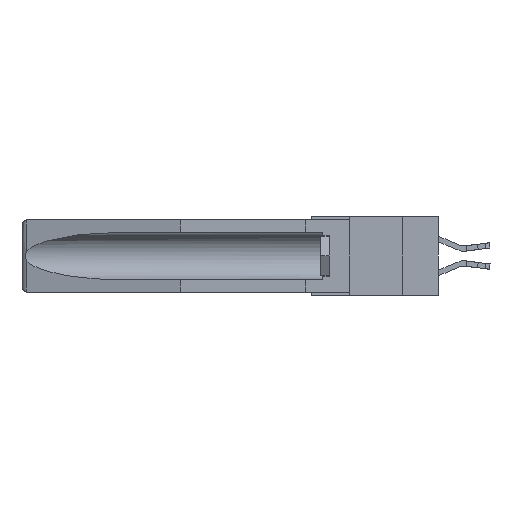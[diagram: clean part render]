
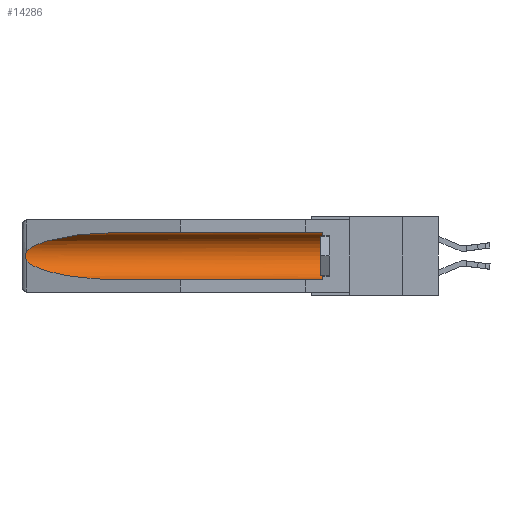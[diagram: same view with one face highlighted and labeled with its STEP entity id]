
A CAD part, left-side view. The second image highlights one B-rep face of the part: STEP entity #14286.
In plain terms, the highlighted cylindrical face has radius 2.857 mm (diameter 5.715 mm), a partial arc.
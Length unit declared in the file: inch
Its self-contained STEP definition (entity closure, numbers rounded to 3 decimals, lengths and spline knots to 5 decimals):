
#65 = LINE ( 'NONE', #9262, #738 ) ;
#738 = VECTOR ( 'NONE', #926, 39.37008 ) ;
#803 = CARTESIAN_POINT ( 'NONE',  ( 0.2673, 1.53269, -0.17917 ) ) ;
#886 = CARTESIAN_POINT ( 'NONE',  ( 0.26654, 1.53092, -0.15636 ) ) ;
#907 = AXIS2_PLACEMENT_3D ( 'NONE', #20044, #23968, #19948 ) ;
#926 = DIRECTION ( 'NONE',  ( 0., 1., 0. ) ) ;
#1354 = VECTOR ( 'NONE', #16719, 39.37008 ) ;
#1902 = CARTESIAN_POINT ( 'NONE',  ( 0.155, -0.30754, -0.284 ) ) ;
#2129 = ORIENTED_EDGE ( 'NONE', *, *, #13327, .T. ) ;
#3458 = CARTESIAN_POINT ( 'NONE',  ( 0.26537, 1.52718, -0.19328 ) ) ;
#3686 = CARTESIAN_POINT ( 'NONE',  ( 0.25451, 1.48313, -0.24835 ) ) ;
#4450 = CARTESIAN_POINT ( 'NONE',  ( 0.155, 1.07973, -0.284 ) ) ;
#4640 = VERTEX_POINT ( 'NONE', #20099 ) ;
#4865 = VERTEX_POINT ( 'NONE', #12742 ) ;
#6241 = EDGE_LOOP ( 'NONE', ( #12499, #10017, #22290, #25767, #2129, #13430 ) ) ;
#6479 = DIRECTION ( 'NONE',  ( 0., 1., 0. ) ) ;
#6636 = VERTEX_POINT ( 'NONE', #12800 ) ;
#6660 = DIRECTION ( 'NONE',  ( 0., 0., 1. ) ) ;
#6828 = CARTESIAN_POINT ( 'NONE',  ( 0.155, 1.07973, -0.059 ) ) ;
#7021 = CARTESIAN_POINT ( 'NONE',  ( 0.26537, 1.52718, -0.14972 ) ) ;
#7631 = VERTEX_POINT ( 'NONE', #4450 ) ;
#7727 = CARTESIAN_POINT ( 'NONE',  ( 0.26537, 1.52718, -0.14972 ) ) ;
#7776 = CARTESIAN_POINT ( 'NONE',  ( 0.21114, 1.30732, -0.284 ) ) ;
#8045 = EDGE_CURVE ( 'NONE', #4865, #6636, #65, .T. ) ;
#9262 = CARTESIAN_POINT ( 'NONE',  ( 0.155, -0.30754, -0.059 ) ) ;
#9271 = FACE_OUTER_BOUND ( 'NONE', #6241, .T. ) ;
#10017 = ORIENTED_EDGE ( 'NONE', *, *, #22010, .T. ) ;
#11835 = CARTESIAN_POINT ( 'NONE',  ( 0.26537, 1.52718, -0.19328 ) ) ;
#12499 = ORIENTED_EDGE ( 'NONE', *, *, #20552, .T. ) ;
#12742 = CARTESIAN_POINT ( 'NONE',  ( 0.155, 0.126, -0.059 ) ) ;
#12800 = CARTESIAN_POINT ( 'NONE',  ( 0.155, 1.07973, -0.059 ) ) ;
#13327 = EDGE_CURVE ( 'NONE', #16865, #4865, #15032, .T. ) ;
#13430 = ORIENTED_EDGE ( 'NONE', *, *, #8045, .T. ) ;
#14097 = CARTESIAN_POINT ( 'NONE',  ( 0.155, 1.07973, -0.284 ) ) ;
#14286 = ADVANCED_FACE ( 'NONE', ( #9271 ), #26576, .F. ) ;
#15032 = CIRCLE ( 'NONE', #907, 0.1125 ) ;
#15741 = LINE ( 'NONE', #1902, #1354 ) ;
#15968 = CARTESIAN_POINT ( 'NONE',  ( 0.26655, 1.53094, -0.18657 ) ) ;
#16456 = CARTESIAN_POINT ( 'NONE',  ( 0.155, 0.126, -0.284 ) ) ;
#16618 =( BOUNDED_CURVE ( )  B_SPLINE_CURVE ( 3, ( #11835, #3686, #7776, #14097 ),
 .UNSPECIFIED., .F., .F. ) 
 B_SPLINE_CURVE_WITH_KNOTS ( ( 4, 4 ),
 ( 0.1948, 1.5708 ),
 .UNSPECIFIED. ) 
 CURVE ( )  GEOMETRIC_REPRESENTATION_ITEM ( )  RATIONAL_B_SPLINE_CURVE ( ( 1., 0.848, 0.848, 1. ) ) 
 REPRESENTATION_ITEM ( '' )  );
#16719 = DIRECTION ( 'NONE',  ( 0., 1., 0. ) ) ;
#16865 = VERTEX_POINT ( 'NONE', #16456 ) ;
#17181 = CARTESIAN_POINT ( 'NONE',  ( 0.21114, 1.30732, -0.059 ) ) ;
#17185 = CARTESIAN_POINT ( 'NONE',  ( 0.155, -0.30754, -0.1715 ) ) ;
#17519 = CARTESIAN_POINT ( 'NONE',  ( 0.2673, 1.5327, -0.16383 ) ) ;
#18147 = CARTESIAN_POINT ( 'NONE',  ( 0.2675, 1.53308, -0.16763 ) ) ;
#19948 = DIRECTION ( 'NONE',  ( 0., 0., 1. ) ) ;
#20044 = CARTESIAN_POINT ( 'NONE',  ( 0.155, 0.126, -0.1715 ) ) ;
#20099 = CARTESIAN_POINT ( 'NONE',  ( 0.26537, 1.52718, -0.19328 ) ) ;
#20542 = AXIS2_PLACEMENT_3D ( 'NONE', #17185, #6479, #6660 ) ;
#20552 = EDGE_CURVE ( 'NONE', #6636, #22657, #24322, .T. ) ;
#21003 = B_SPLINE_CURVE_WITH_KNOTS ( 'NONE', 3,
 ( #7727, #26560, #886, #17519, #18147, #22372, #803, #15968, #21762, #3458 ),
 .UNSPECIFIED., .F., .F.,
 ( 4, 2, 2, 2, 4 ),
 ( 0., 0.00029, 0.00058, 0.00087, 0.00117 ),
 .UNSPECIFIED. ) ;
#21395 = CARTESIAN_POINT ( 'NONE',  ( 0.25451, 1.48313, -0.09465 ) ) ;
#21762 = CARTESIAN_POINT ( 'NONE',  ( 0.26597, 1.5296, -0.19026 ) ) ;
#22010 = EDGE_CURVE ( 'NONE', #22657, #4640, #21003, .T. ) ;
#22290 = ORIENTED_EDGE ( 'NONE', *, *, #23983, .T. ) ;
#22372 = CARTESIAN_POINT ( 'NONE',  ( 0.2675, 1.53308, -0.17534 ) ) ;
#22657 = VERTEX_POINT ( 'NONE', #25515 ) ;
#23968 = DIRECTION ( 'NONE',  ( 0., -1., 0. ) ) ;
#23983 = EDGE_CURVE ( 'NONE', #4640, #7631, #16618, .T. ) ;
#24322 =( BOUNDED_CURVE ( )  B_SPLINE_CURVE ( 3, ( #6828, #17181, #21395, #7021 ),
 .UNSPECIFIED., .F., .F. ) 
 B_SPLINE_CURVE_WITH_KNOTS ( ( 4, 4 ),
 ( 4.71239, 6.08839 ),
 .UNSPECIFIED. ) 
 CURVE ( )  GEOMETRIC_REPRESENTATION_ITEM ( )  RATIONAL_B_SPLINE_CURVE ( ( 1., 0.848, 0.848, 1. ) ) 
 REPRESENTATION_ITEM ( '' )  );
#24408 = EDGE_CURVE ( 'NONE', #16865, #7631, #15741, .T. ) ;
#25515 = CARTESIAN_POINT ( 'NONE',  ( 0.26537, 1.52718, -0.14972 ) ) ;
#25767 = ORIENTED_EDGE ( 'NONE', *, *, #24408, .F. ) ;
#26560 = CARTESIAN_POINT ( 'NONE',  ( 0.26597, 1.52961, -0.15275 ) ) ;
#26576 = CYLINDRICAL_SURFACE ( 'NONE', #20542, 0.1125 ) ;
